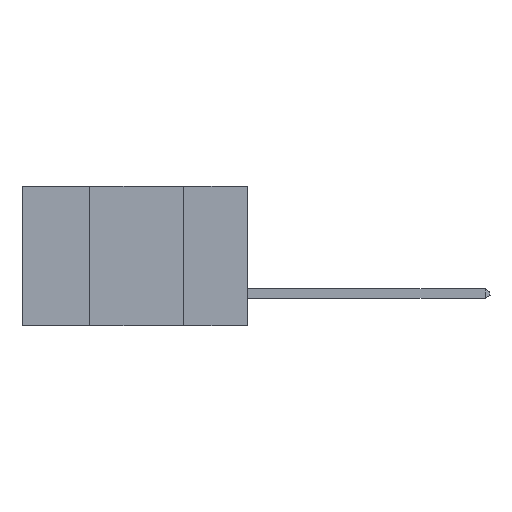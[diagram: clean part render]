
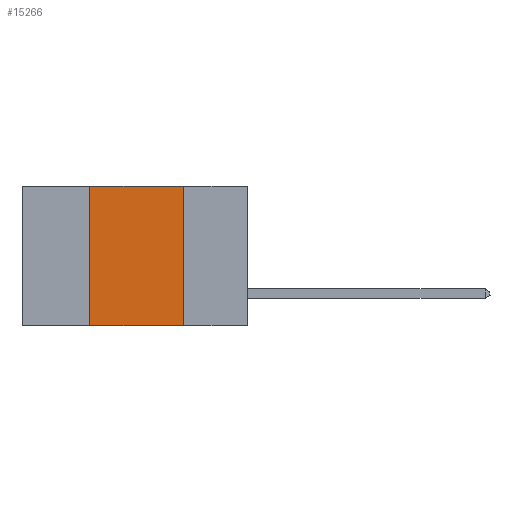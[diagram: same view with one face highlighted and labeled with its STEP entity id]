
A CAD part, left-side view. The second image highlights one B-rep face of the part: STEP entity #15266.
In plain terms, the highlighted planar face has unit normal (-1, 0, 0).
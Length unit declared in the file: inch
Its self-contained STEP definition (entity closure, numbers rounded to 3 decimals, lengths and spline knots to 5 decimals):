
#631 = ORIENTED_EDGE ( 'NONE', *, *, #8781, .F. ) ;
#946 = VECTOR ( 'NONE', #4035, 39.37008 ) ;
#2935 = LINE ( 'NONE', #14077, #8072 ) ;
#3811 = CARTESIAN_POINT ( 'NONE',  ( 0., 0.17, -0.37 ) ) ;
#4035 = DIRECTION ( 'NONE',  ( 0., -1., 0. ) ) ;
#4631 = LINE ( 'NONE', #12612, #946 ) ;
#4694 = VERTEX_POINT ( 'NONE', #15674 ) ;
#4862 = DIRECTION ( 'NONE',  ( 0., 0., -1. ) ) ;
#5141 = FACE_OUTER_BOUND ( 'NONE', #8461, .T. ) ;
#6078 = CARTESIAN_POINT ( 'NONE',  ( 0., 0.42, 0. ) ) ;
#6303 = PLANE ( 'NONE',  #15147 ) ;
#6444 = DIRECTION ( 'NONE',  ( 0., 0., 1. ) ) ;
#7226 = CARTESIAN_POINT ( 'NONE',  ( 0., 0.42, -0.37 ) ) ;
#7344 = EDGE_CURVE ( 'NONE', #16145, #11374, #14233, .T. ) ;
#7370 = ORIENTED_EDGE ( 'NONE', *, *, #10306, .F. ) ;
#7975 = VERTEX_POINT ( 'NONE', #3811 ) ;
#8026 = EDGE_CURVE ( 'NONE', #16145, #7975, #11757, .T. ) ;
#8072 = VECTOR ( 'NONE', #11037, 39.37008 ) ;
#8461 = EDGE_LOOP ( 'NONE', ( #631, #7370, #10990, #13456 ) ) ;
#8781 = EDGE_CURVE ( 'NONE', #4694, #7975, #2935, .T. ) ;
#8815 = CARTESIAN_POINT ( 'NONE',  ( 0., 0.42, 0. ) ) ;
#9157 = CARTESIAN_POINT ( 'NONE',  ( 0., 0.6, -0.37 ) ) ;
#9897 = VECTOR ( 'NONE', #6444, 39.37008 ) ;
#10306 = EDGE_CURVE ( 'NONE', #11374, #4694, #4631, .T. ) ;
#10903 = VECTOR ( 'NONE', #17712, 39.37008 ) ;
#10990 = ORIENTED_EDGE ( 'NONE', *, *, #7344, .F. ) ;
#11037 = DIRECTION ( 'NONE',  ( 0., 0., -1. ) ) ;
#11374 = VERTEX_POINT ( 'NONE', #8815 ) ;
#11757 = LINE ( 'NONE', #9157, #10903 ) ;
#11868 = CARTESIAN_POINT ( 'NONE',  ( 0., 0.6, 0. ) ) ;
#12612 = CARTESIAN_POINT ( 'NONE',  ( 0., 0.6, 0. ) ) ;
#13456 = ORIENTED_EDGE ( 'NONE', *, *, #8026, .T. ) ;
#14077 = CARTESIAN_POINT ( 'NONE',  ( 0., 0.17, 0. ) ) ;
#14233 = LINE ( 'NONE', #6078, #9897 ) ;
#15147 = AXIS2_PLACEMENT_3D ( 'NONE', #11868, #15982, #4862 ) ;
#15266 = ADVANCED_FACE ( 'NONE', ( #5141 ), #6303, .F. ) ;
#15674 = CARTESIAN_POINT ( 'NONE',  ( 0., 0.17, 0. ) ) ;
#15982 = DIRECTION ( 'NONE',  ( 1., 0., 0. ) ) ;
#16145 = VERTEX_POINT ( 'NONE', #7226 ) ;
#17712 = DIRECTION ( 'NONE',  ( 0., -1., 0. ) ) ;
